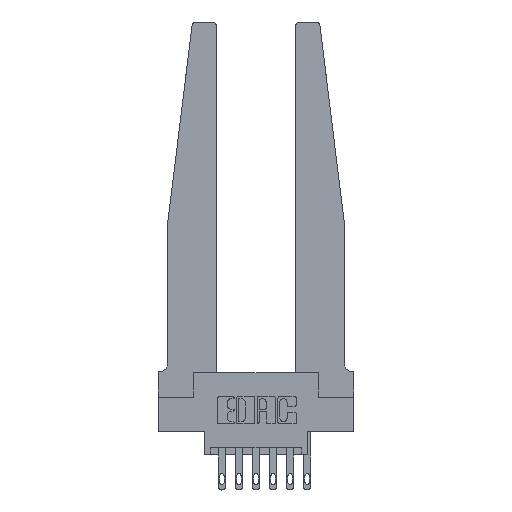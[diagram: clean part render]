
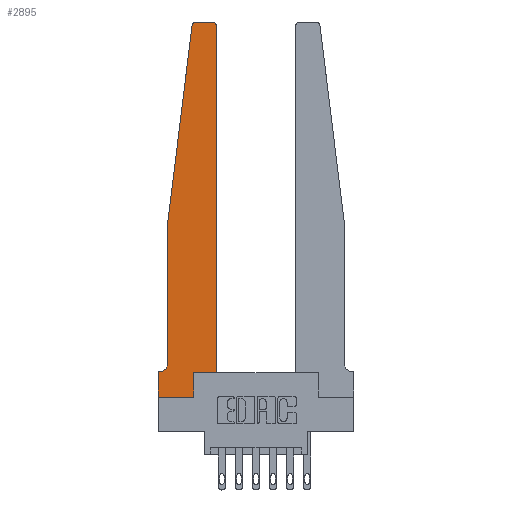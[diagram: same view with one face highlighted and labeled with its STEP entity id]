
A CAD part, top view. The second image highlights one B-rep face of the part: STEP entity #2895.
In plain terms, the highlighted planar face has unit normal (0, 0, 1).
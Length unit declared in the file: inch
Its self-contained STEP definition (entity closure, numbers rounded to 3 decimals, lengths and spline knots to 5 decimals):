
#206 = DIRECTION ( 'NONE',  ( -1., 0., 0. ) ) ;
#230 = VERTEX_POINT ( 'NONE', #9587 ) ;
#527 = VERTEX_POINT ( 'NONE', #5377 ) ;
#602 = CARTESIAN_POINT ( 'NONE',  ( 0.24675, 2.72367, 0.37 ) ) ;
#692 = CARTESIAN_POINT ( 'NONE',  ( 0.2605, 0.18, 0.37 ) ) ;
#906 = AXIS2_PLACEMENT_3D ( 'NONE', #12334, #2919, #13240 ) ;
#1260 = LINE ( 'NONE', #7493, #8881 ) ;
#1416 = DIRECTION ( 'NONE',  ( 0., 1., 0. ) ) ;
#1439 = DIRECTION ( 'NONE',  ( 1., 0., 0. ) ) ;
#1480 = EDGE_CURVE ( 'NONE', #527, #12855, #7419, .T. ) ;
#1485 = DIRECTION ( 'NONE',  ( 0., -1., 0. ) ) ;
#1491 = LINE ( 'NONE', #1561, #11292 ) ;
#1561 = CARTESIAN_POINT ( 'NONE',  ( 0.2605, 0.18, 0.37 ) ) ;
#1614 = LINE ( 'NONE', #2703, #7794 ) ;
#1688 = LINE ( 'NONE', #10200, #5467 ) ;
#1712 = EDGE_CURVE ( 'NONE', #2813, #7674, #1688, .T. ) ;
#1752 = DIRECTION ( 'NONE',  ( 1., 0., 0. ) ) ;
#2164 = VERTEX_POINT ( 'NONE', #6045 ) ;
#2299 = CIRCLE ( 'NONE', #7554, 0.03 ) ;
#2373 = DIRECTION ( 'NONE',  ( -0.122, -0.992, 0. ) ) ;
#2639 = ORIENTED_EDGE ( 'NONE', *, *, #8350, .T. ) ;
#2640 = ORIENTED_EDGE ( 'NONE', *, *, #7112, .T. ) ;
#2703 = CARTESIAN_POINT ( 'NONE',  ( 0.425, 0.18, 0.37 ) ) ;
#2813 = VERTEX_POINT ( 'NONE', #9810 ) ;
#2895 = ADVANCED_FACE ( 'NONE', ( #3478 ), #11864, .T. ) ;
#2919 = DIRECTION ( 'NONE',  ( 0., 0., -1. ) ) ;
#3033 = CARTESIAN_POINT ( 'NONE',  ( 0., 0., 0.37 ) ) ;
#3478 = FACE_OUTER_BOUND ( 'NONE', #10082, .T. ) ;
#3489 = CIRCLE ( 'NONE', #4156, 0.03 ) ;
#3597 = VECTOR ( 'NONE', #2373, 39.37008 ) ;
#3678 = VERTEX_POINT ( 'NONE', #13064 ) ;
#3710 = CARTESIAN_POINT ( 'NONE',  ( 0.065, 0.2375, 0.37 ) ) ;
#3937 = DIRECTION ( 'NONE',  ( 1., 0., 0. ) ) ;
#4055 = DIRECTION ( 'NONE',  ( 0., -1., 0. ) ) ;
#4067 = DIRECTION ( 'NONE',  ( -1., 0., 0. ) ) ;
#4072 = DIRECTION ( 'NONE',  ( 1., 0., 0. ) ) ;
#4156 = AXIS2_PLACEMENT_3D ( 'NONE', #8148, #5938, #4072 ) ;
#4261 = CARTESIAN_POINT ( 'NONE',  ( 0., 0.1875, 0.37 ) ) ;
#4564 = ORIENTED_EDGE ( 'NONE', *, *, #4768, .T. ) ;
#4768 = EDGE_CURVE ( 'NONE', #12855, #2164, #8566, .T. ) ;
#4783 = ORIENTED_EDGE ( 'NONE', *, *, #1712, .T. ) ;
#4864 = ORIENTED_EDGE ( 'NONE', *, *, #10640, .T. ) ;
#5185 = LINE ( 'NONE', #11424, #6616 ) ;
#5263 = CARTESIAN_POINT ( 'NONE',  ( 0.425, 0.18, 0.37 ) ) ;
#5358 = ORIENTED_EDGE ( 'NONE', *, *, #6087, .T. ) ;
#5377 = CARTESIAN_POINT ( 'NONE',  ( 0.065, 1.25, 0.37 ) ) ;
#5467 = VECTOR ( 'NONE', #1752, 39.37008 ) ;
#5490 = DIRECTION ( 'NONE',  ( 1., 0., 0. ) ) ;
#5659 = CARTESIAN_POINT ( 'NONE',  ( 0.065, 1.25, 0.37 ) ) ;
#5709 = CARTESIAN_POINT ( 'NONE',  ( 0.425, 0.18, 0.37 ) ) ;
#5938 = DIRECTION ( 'NONE',  ( 0., 0., 1. ) ) ;
#6045 = CARTESIAN_POINT ( 'NONE',  ( 0.015, 0.1875, 0.37 ) ) ;
#6087 = EDGE_CURVE ( 'NONE', #3678, #13502, #3489, .T. ) ;
#6616 = VECTOR ( 'NONE', #4067, 39.37008 ) ;
#6638 = DIRECTION ( 'NONE',  ( 0., 0., 1. ) ) ;
#6770 = VERTEX_POINT ( 'NONE', #5709 ) ;
#6853 = ORIENTED_EDGE ( 'NONE', *, *, #12003, .T. ) ;
#7112 = EDGE_CURVE ( 'NONE', #10764, #6770, #8347, .T. ) ;
#7258 = VECTOR ( 'NONE', #3937, 39.37008 ) ;
#7419 = LINE ( 'NONE', #5659, #12914 ) ;
#7463 = CARTESIAN_POINT ( 'NONE',  ( 0.065, 1.25, 0.37 ) ) ;
#7493 = CARTESIAN_POINT ( 'NONE',  ( 0.065, 0.1875, 0.37 ) ) ;
#7554 = AXIS2_PLACEMENT_3D ( 'NONE', #12707, #12912, #5490 ) ;
#7674 = VERTEX_POINT ( 'NONE', #9638 ) ;
#7794 = VECTOR ( 'NONE', #1416, 39.37008 ) ;
#8148 = CARTESIAN_POINT ( 'NONE',  ( 0.27653, 2.72, 0.37 ) ) ;
#8347 = LINE ( 'NONE', #5263, #7258 ) ;
#8350 = EDGE_CURVE ( 'NONE', #230, #3678, #5185, .T. ) ;
#8353 = ORIENTED_EDGE ( 'NONE', *, *, #8716, .T. ) ;
#8437 = ORIENTED_EDGE ( 'NONE', *, *, #11451, .T. ) ;
#8566 = CIRCLE ( 'NONE', #906, 0.05 ) ;
#8716 = EDGE_CURVE ( 'NONE', #11842, #2813, #13357, .T. ) ;
#8881 = VECTOR ( 'NONE', #206, 39.37008 ) ;
#8966 = CARTESIAN_POINT ( 'NONE',  ( 0., 0.1875, 0.37 ) ) ;
#9017 = ORIENTED_EDGE ( 'NONE', *, *, #13386, .T. ) ;
#9034 = VERTEX_POINT ( 'NONE', #10989 ) ;
#9413 = ORIENTED_EDGE ( 'NONE', *, *, #1480, .T. ) ;
#9587 = CARTESIAN_POINT ( 'NONE',  ( 0.395, 2.75, 0.37 ) ) ;
#9638 = CARTESIAN_POINT ( 'NONE',  ( 0.2605, 0., 0.37 ) ) ;
#9810 = CARTESIAN_POINT ( 'NONE',  ( 0., 0., 0.37 ) ) ;
#10082 = EDGE_LOOP ( 'NONE', ( #2639, #5358, #8437, #9413, #4564, #6853, #8353, #4783, #9017, #2640, #10402, #4864 ) ) ;
#10200 = CARTESIAN_POINT ( 'NONE',  ( 0., 0., 0.37 ) ) ;
#10402 = ORIENTED_EDGE ( 'NONE', *, *, #11552, .T. ) ;
#10446 = LINE ( 'NONE', #7463, #3597 ) ;
#10640 = EDGE_CURVE ( 'NONE', #9034, #230, #2299, .T. ) ;
#10691 = DIRECTION ( 'NONE',  ( 0., 1., 0. ) ) ;
#10764 = VERTEX_POINT ( 'NONE', #692 ) ;
#10989 = CARTESIAN_POINT ( 'NONE',  ( 0.425, 2.72, 0.37 ) ) ;
#11292 = VECTOR ( 'NONE', #10691, 39.37008 ) ;
#11424 = CARTESIAN_POINT ( 'NONE',  ( 0.25, 2.75, 0.37 ) ) ;
#11451 = EDGE_CURVE ( 'NONE', #13502, #527, #10446, .T. ) ;
#11552 = EDGE_CURVE ( 'NONE', #6770, #9034, #1614, .T. ) ;
#11674 = VECTOR ( 'NONE', #4055, 39.37008 ) ;
#11842 = VERTEX_POINT ( 'NONE', #4261 ) ;
#11864 = PLANE ( 'NONE',  #12534 ) ;
#12003 = EDGE_CURVE ( 'NONE', #2164, #11842, #1260, .T. ) ;
#12334 = CARTESIAN_POINT ( 'NONE',  ( 0.015, 0.2375, 0.37 ) ) ;
#12534 = AXIS2_PLACEMENT_3D ( 'NONE', #8966, #6638, #1439 ) ;
#12707 = CARTESIAN_POINT ( 'NONE',  ( 0.395, 2.72, 0.37 ) ) ;
#12855 = VERTEX_POINT ( 'NONE', #3710 ) ;
#12912 = DIRECTION ( 'NONE',  ( 0., 0., 1. ) ) ;
#12914 = VECTOR ( 'NONE', #1485, 39.37008 ) ;
#13064 = CARTESIAN_POINT ( 'NONE',  ( 0.27653, 2.75, 0.37 ) ) ;
#13240 = DIRECTION ( 'NONE',  ( -1., 0., 0. ) ) ;
#13357 = LINE ( 'NONE', #3033, #11674 ) ;
#13386 = EDGE_CURVE ( 'NONE', #7674, #10764, #1491, .T. ) ;
#13502 = VERTEX_POINT ( 'NONE', #602 ) ;
